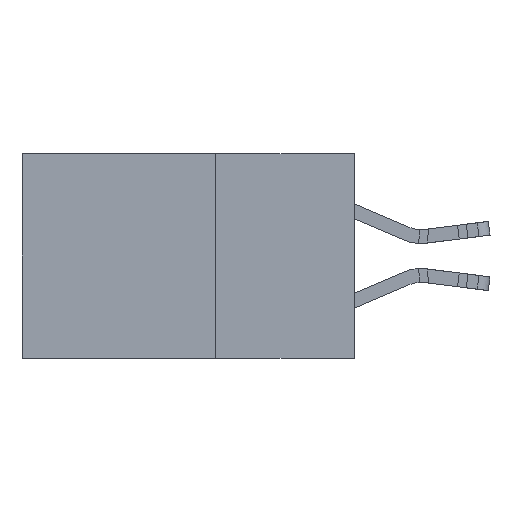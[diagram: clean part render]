
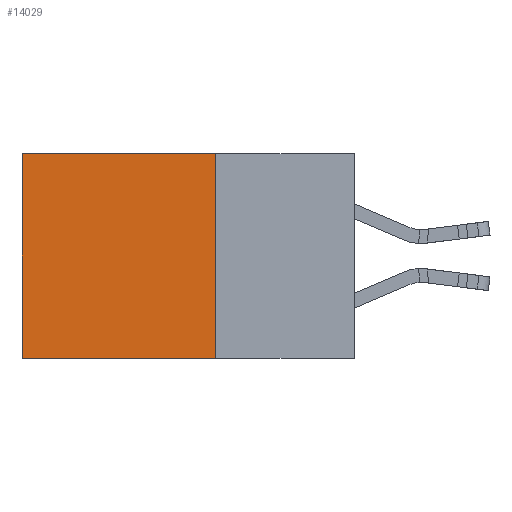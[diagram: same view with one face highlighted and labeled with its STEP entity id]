
A CAD part, left-side view. The second image highlights one B-rep face of the part: STEP entity #14029.
In plain terms, the highlighted planar face has unit normal (-1, 0, 0).
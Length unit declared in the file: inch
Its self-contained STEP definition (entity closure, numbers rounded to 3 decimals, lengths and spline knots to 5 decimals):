
#230 = VECTOR ( 'NONE', #21029, 39.37008 ) ;
#456 = CARTESIAN_POINT ( 'NONE',  ( 0.298, 0.25, 0. ) ) ;
#849 = VERTEX_POINT ( 'NONE', #10055 ) ;
#2083 = VERTEX_POINT ( 'NONE', #19315 ) ;
#2324 = DIRECTION ( 'NONE',  ( 0., 1., 0. ) ) ;
#2715 = FACE_OUTER_BOUND ( 'NONE', #12911, .T. ) ;
#2760 = DIRECTION ( 'NONE',  ( 1., 0., 0. ) ) ;
#5513 = LINE ( 'NONE', #28335, #17087 ) ;
#6167 = VERTEX_POINT ( 'NONE', #7661 ) ;
#6869 = VECTOR ( 'NONE', #26309, 39.37008 ) ;
#7661 = CARTESIAN_POINT ( 'NONE',  ( 0.298, 0.6, 0. ) ) ;
#7729 = EDGE_CURVE ( 'NONE', #2083, #849, #16533, .T. ) ;
#7885 = LINE ( 'NONE', #11922, #230 ) ;
#10055 = CARTESIAN_POINT ( 'NONE',  ( 0.298, 0.6, -0.37 ) ) ;
#10938 = ORIENTED_EDGE ( 'NONE', *, *, #7729, .F. ) ;
#11618 = CARTESIAN_POINT ( 'NONE',  ( 0.298, 0.25, -0.37 ) ) ;
#11922 = CARTESIAN_POINT ( 'NONE',  ( 0.298, 0.25, 0. ) ) ;
#12669 = CARTESIAN_POINT ( 'NONE',  ( 0.298, 0.25, 0. ) ) ;
#12911 = EDGE_LOOP ( 'NONE', ( #27968, #10938, #20725, #27801 ) ) ;
#13739 = LINE ( 'NONE', #12669, #6869 ) ;
#13872 = VERTEX_POINT ( 'NONE', #20664 ) ;
#14029 = ADVANCED_FACE ( 'NONE', ( #2715 ), #16658, .F. ) ;
#16101 = EDGE_CURVE ( 'NONE', #6167, #849, #5513, .T. ) ;
#16533 = LINE ( 'NONE', #11618, #27883 ) ;
#16658 = PLANE ( 'NONE',  #26690 ) ;
#17087 = VECTOR ( 'NONE', #23929, 39.37008 ) ;
#18933 = DIRECTION ( 'NONE',  ( 0., 0., -1. ) ) ;
#19315 = CARTESIAN_POINT ( 'NONE',  ( 0.298, 0.25, -0.37 ) ) ;
#20664 = CARTESIAN_POINT ( 'NONE',  ( 0.298, 0.25, 0. ) ) ;
#20725 = ORIENTED_EDGE ( 'NONE', *, *, #26205, .F. ) ;
#21029 = DIRECTION ( 'NONE',  ( 0., 1., 0. ) ) ;
#23929 = DIRECTION ( 'NONE',  ( 0., 0., -1. ) ) ;
#26205 = EDGE_CURVE ( 'NONE', #13872, #2083, #13739, .T. ) ;
#26309 = DIRECTION ( 'NONE',  ( 0., 0., -1. ) ) ;
#26690 = AXIS2_PLACEMENT_3D ( 'NONE', #456, #2760, #18933 ) ;
#27349 = EDGE_CURVE ( 'NONE', #13872, #6167, #7885, .T. ) ;
#27801 = ORIENTED_EDGE ( 'NONE', *, *, #27349, .T. ) ;
#27883 = VECTOR ( 'NONE', #2324, 39.37008 ) ;
#27968 = ORIENTED_EDGE ( 'NONE', *, *, #16101, .T. ) ;
#28335 = CARTESIAN_POINT ( 'NONE',  ( 0.298, 0.6, 0. ) ) ;
